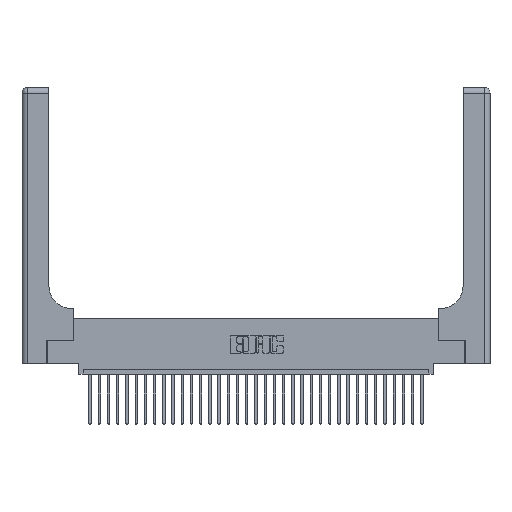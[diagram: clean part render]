
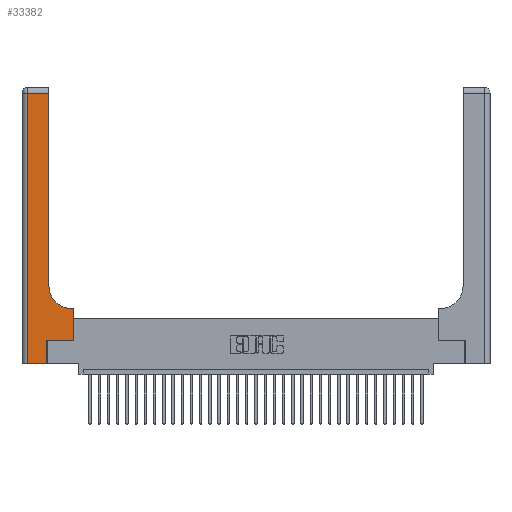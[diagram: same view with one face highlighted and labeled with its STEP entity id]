
A CAD part, top view. The second image highlights one B-rep face of the part: STEP entity #33382.
In plain terms, the highlighted planar face has unit normal (0, 0, 1).
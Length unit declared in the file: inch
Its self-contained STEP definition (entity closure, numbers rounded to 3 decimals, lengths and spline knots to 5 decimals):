
#65 = DIRECTION ( 'NONE',  ( -1., 0., 0. ) ) ;
#569 = CARTESIAN_POINT ( 'NONE',  ( 0.2915, 0.6, 0.37 ) ) ;
#889 = VECTOR ( 'NONE', #11469, 39.37008 ) ;
#1002 = EDGE_CURVE ( 'NONE', #9409, #20841, #9243, .T. ) ;
#1198 = VERTEX_POINT ( 'NONE', #12535 ) ;
#1342 = LINE ( 'NONE', #4245, #3336 ) ;
#3336 = VECTOR ( 'NONE', #14261, 39.37008 ) ;
#3809 = AXIS2_PLACEMENT_3D ( 'NONE', #31616, #10615, #65 ) ;
#4245 = CARTESIAN_POINT ( 'NONE',  ( 0., 0., 0.37 ) ) ;
#4676 = ORIENTED_EDGE ( 'NONE', *, *, #16488, .T. ) ;
#5098 = CARTESIAN_POINT ( 'NONE',  ( 0.5415, 0.6, 0.37 ) ) ;
#5794 = CARTESIAN_POINT ( 'NONE',  ( 0.06, 3., 0.37 ) ) ;
#6372 = DIRECTION ( 'NONE',  ( 0., 0., -1. ) ) ;
#6630 = ORIENTED_EDGE ( 'NONE', *, *, #7824, .T. ) ;
#7220 = FACE_OUTER_BOUND ( 'NONE', #8605, .T. ) ;
#7331 = CARTESIAN_POINT ( 'NONE',  ( 0.269, 0., 0.37 ) ) ;
#7476 = VECTOR ( 'NONE', #18683, 39.37008 ) ;
#7824 = EDGE_CURVE ( 'NONE', #20841, #21989, #31634, .T. ) ;
#8326 = EDGE_CURVE ( 'NONE', #15460, #1198, #8998, .T. ) ;
#8605 = EDGE_LOOP ( 'NONE', ( #13380, #4676, #13215, #23904, #16399, #23920, #11940, #6630, #24127 ) ) ;
#8998 = LINE ( 'NONE', #7331, #889 ) ;
#9243 = LINE ( 'NONE', #14368, #16181 ) ;
#9409 = VERTEX_POINT ( 'NONE', #19374 ) ;
#9481 = EDGE_CURVE ( 'NONE', #21989, #19875, #17081, .T. ) ;
#10615 = DIRECTION ( 'NONE',  ( 0., 0., -1. ) ) ;
#11469 = DIRECTION ( 'NONE',  ( 0., 1., 0. ) ) ;
#11547 = VECTOR ( 'NONE', #28798, 39.37008 ) ;
#11738 = VERTEX_POINT ( 'NONE', #12262 ) ;
#11940 = ORIENTED_EDGE ( 'NONE', *, *, #1002, .T. ) ;
#12262 = CARTESIAN_POINT ( 'NONE',  ( 0.2915, 2.94, 0.37 ) ) ;
#12292 = DIRECTION ( 'NONE',  ( 0., 1., 0. ) ) ;
#12330 = LINE ( 'NONE', #22900, #32433 ) ;
#12465 = AXIS2_PLACEMENT_3D ( 'NONE', #14119, #6372, #26905 ) ;
#12535 = CARTESIAN_POINT ( 'NONE',  ( 0.269, 0.25, 0.37 ) ) ;
#12945 = LINE ( 'NONE', #5794, #23156 ) ;
#13215 = ORIENTED_EDGE ( 'NONE', *, *, #23725, .T. ) ;
#13380 = ORIENTED_EDGE ( 'NONE', *, *, #14028, .T. ) ;
#14028 = EDGE_CURVE ( 'NONE', #19875, #11738, #12330, .T. ) ;
#14119 = CARTESIAN_POINT ( 'NONE',  ( 0.5415, 0.85, 0.37 ) ) ;
#14261 = DIRECTION ( 'NONE',  ( 1., 0., 0. ) ) ;
#14368 = CARTESIAN_POINT ( 'NONE',  ( 0.5585, 0.25, 0.37 ) ) ;
#15200 = CARTESIAN_POINT ( 'NONE',  ( 0.06, 0., 0.37 ) ) ;
#15235 = LINE ( 'NONE', #23496, #11547 ) ;
#15460 = VERTEX_POINT ( 'NONE', #18635 ) ;
#15723 = DIRECTION ( 'NONE',  ( 0., -1., 0. ) ) ;
#16004 = PLANE ( 'NONE',  #3809 ) ;
#16181 = VECTOR ( 'NONE', #33506, 39.37008 ) ;
#16399 = ORIENTED_EDGE ( 'NONE', *, *, #8326, .T. ) ;
#16488 = EDGE_CURVE ( 'NONE', #11738, #31123, #15235, .T. ) ;
#17081 = CIRCLE ( 'NONE', #12465, 0.25 ) ;
#17272 = CARTESIAN_POINT ( 'NONE',  ( 0.2915, 0.85, 0.37 ) ) ;
#18629 = VECTOR ( 'NONE', #25373, 39.37008 ) ;
#18635 = CARTESIAN_POINT ( 'NONE',  ( 0.269, 0., 0.37 ) ) ;
#18683 = DIRECTION ( 'NONE',  ( -1., 0., 0. ) ) ;
#19374 = CARTESIAN_POINT ( 'NONE',  ( 0.5585, 0.25, 0.37 ) ) ;
#19875 = VERTEX_POINT ( 'NONE', #17272 ) ;
#20841 = VERTEX_POINT ( 'NONE', #26118 ) ;
#21094 = EDGE_CURVE ( 'NONE', #26205, #15460, #1342, .T. ) ;
#21989 = VERTEX_POINT ( 'NONE', #5098 ) ;
#22900 = CARTESIAN_POINT ( 'NONE',  ( 0.2915, 3., 0.37 ) ) ;
#23156 = VECTOR ( 'NONE', #15723, 39.37008 ) ;
#23496 = CARTESIAN_POINT ( 'NONE',  ( 0., 2.94, 0.37 ) ) ;
#23725 = EDGE_CURVE ( 'NONE', #31123, #26205, #12945, .T. ) ;
#23904 = ORIENTED_EDGE ( 'NONE', *, *, #21094, .T. ) ;
#23920 = ORIENTED_EDGE ( 'NONE', *, *, #26130, .T. ) ;
#24127 = ORIENTED_EDGE ( 'NONE', *, *, #9481, .T. ) ;
#25258 = CARTESIAN_POINT ( 'NONE',  ( 0.06, 2.94, 0.37 ) ) ;
#25373 = DIRECTION ( 'NONE',  ( 1., 0., 0. ) ) ;
#25704 = CARTESIAN_POINT ( 'NONE',  ( 0.269, 0.25, 0.37 ) ) ;
#26118 = CARTESIAN_POINT ( 'NONE',  ( 0.5585, 0.6, 0.37 ) ) ;
#26130 = EDGE_CURVE ( 'NONE', #1198, #9409, #32635, .T. ) ;
#26205 = VERTEX_POINT ( 'NONE', #15200 ) ;
#26905 = DIRECTION ( 'NONE',  ( 1., 0., 0. ) ) ;
#28798 = DIRECTION ( 'NONE',  ( -1., 0., 0. ) ) ;
#31123 = VERTEX_POINT ( 'NONE', #25258 ) ;
#31616 = CARTESIAN_POINT ( 'NONE',  ( 0., 3., 0.37 ) ) ;
#31634 = LINE ( 'NONE', #569, #7476 ) ;
#32433 = VECTOR ( 'NONE', #12292, 39.37008 ) ;
#32635 = LINE ( 'NONE', #25704, #18629 ) ;
#33382 = ADVANCED_FACE ( 'NONE', ( #7220 ), #16004, .F. ) ;
#33506 = DIRECTION ( 'NONE',  ( 0., 1., 0. ) ) ;
